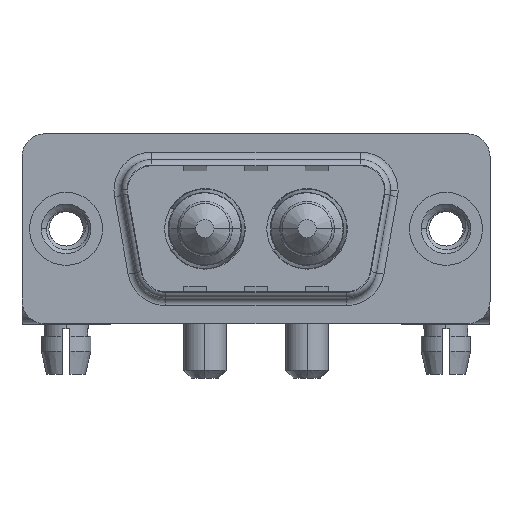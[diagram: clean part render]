
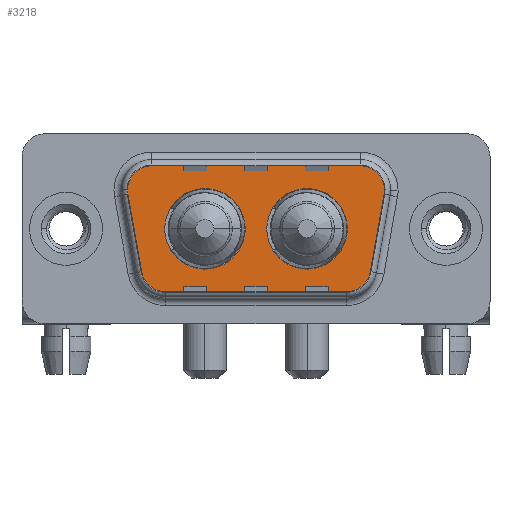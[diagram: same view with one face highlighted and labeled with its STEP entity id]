
A CAD part, top view. The second image highlights one B-rep face of the part: STEP entity #3218.
In plain terms, the highlighted planar face has unit normal (0, 0, 1).
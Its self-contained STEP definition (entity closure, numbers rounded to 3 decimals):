
#93 = ORIENTED_EDGE ( 'NONE', *, *, #6809, .T. ) ;
#292 = EDGE_CURVE ( 'NONE', #4392, #8052, #645, .T. ) ;
#318 = VECTOR ( 'NONE', #12511, 1000. ) ;
#425 = AXIS2_PLACEMENT_3D ( 'NONE', #1729, #8569, #3206 ) ;
#520 = EDGE_CURVE ( 'NONE', #8263, #11774, #11003, .T. ) ;
#546 = CARTESIAN_POINT ( 'NONE',  ( 6.459, -4.9, 0. ) ) ;
#645 = CIRCLE ( 'NONE', #7865, 2. ) ;
#710 = CARTESIAN_POINT ( 'NONE',  ( 19.564, 4.9, 0. ) ) ;
#712 = CARTESIAN_POINT ( 'NONE',  ( 5.436, 4.9, 0. ) ) ;
#745 = DIRECTION ( 'NONE',  ( 0., 0., 1. ) ) ;
#766 = AXIS2_PLACEMENT_3D ( 'NONE', #2552, #10178, #11172 ) ;
#946 = DIRECTION ( 'NONE',  ( 1., 0., 0. ) ) ;
#958 = CARTESIAN_POINT ( 'NONE',  ( 3.466, 2.553, 0. ) ) ;
#1144 = AXIS2_PLACEMENT_3D ( 'NONE', #13453, #7114, #12419 ) ;
#1146 = VECTOR ( 'NONE', #11630, 1000. ) ;
#1548 = CIRCLE ( 'NONE', #425, 2.65 ) ;
#1671 = DIRECTION ( 'NONE',  ( -1., 0., 0. ) ) ;
#1729 = CARTESIAN_POINT ( 'NONE',  ( 9.14, 0., 0. ) ) ;
#2175 = DIRECTION ( 'NONE',  ( 0.174, 0.985, 0. ) ) ;
#2304 = CARTESIAN_POINT ( 'NONE',  ( 21.564, 2.9, 0. ) ) ;
#2376 = LINE ( 'NONE', #5750, #10346 ) ;
#2386 = LINE ( 'NONE', #6473, #11758 ) ;
#2420 = ORIENTED_EDGE ( 'NONE', *, *, #4093, .F. ) ;
#2552 = CARTESIAN_POINT ( 'NONE',  ( 19.564, 2.9, 0. ) ) ;
#2633 = EDGE_LOOP ( 'NONE', ( #11401, #3628 ) ) ;
#3144 = AXIS2_PLACEMENT_3D ( 'NONE', #7506, #10627, #946 ) ;
#3206 = DIRECTION ( 'NONE',  ( 1., 0., 0. ) ) ;
#3218 = ADVANCED_FACE ( 'NONE', ( #9604, #5371, #6571 ), #3320, .T. ) ;
#3296 = CARTESIAN_POINT ( 'NONE',  ( 19.564, 2.9, 0. ) ) ;
#3320 = PLANE ( 'NONE',  #8345 ) ;
#3398 = DIRECTION ( 'NONE',  ( 0., 0., 1. ) ) ;
#3628 = ORIENTED_EDGE ( 'NONE', *, *, #4674, .F. ) ;
#3657 = EDGE_CURVE ( 'NONE', #7756, #6513, #9692, .T. ) ;
#3659 = ORIENTED_EDGE ( 'NONE', *, *, #520, .T. ) ;
#3687 = LINE ( 'NONE', #712, #318 ) ;
#3720 = ORIENTED_EDGE ( 'NONE', *, *, #6664, .T. ) ;
#3819 = ORIENTED_EDGE ( 'NONE', *, *, #4346, .T. ) ;
#4093 = EDGE_CURVE ( 'NONE', #10286, #13687, #13532, .T. ) ;
#4158 = DIRECTION ( 'NONE',  ( 0., 0., 1. ) ) ;
#4346 = EDGE_CURVE ( 'NONE', #11774, #12296, #2376, .T. ) ;
#4392 = VERTEX_POINT ( 'NONE', #2304 ) ;
#4395 = CARTESIAN_POINT ( 'NONE',  ( 5.436, 4.9, 0. ) ) ;
#4599 = EDGE_CURVE ( 'NONE', #6779, #8497, #1548, .T. ) ;
#4674 = EDGE_CURVE ( 'NONE', #8497, #6779, #7204, .T. ) ;
#5371 = FACE_BOUND ( 'NONE', #2633, .T. ) ;
#5428 = CARTESIAN_POINT ( 'NONE',  ( 15.86, 0., 0. ) ) ;
#5509 = CARTESIAN_POINT ( 'NONE',  ( 18.541, -2.9, 0. ) ) ;
#5637 = EDGE_CURVE ( 'NONE', #12296, #7199, #6050, .T. ) ;
#5750 = CARTESIAN_POINT ( 'NONE',  ( 6.459, -4.9, 0. ) ) ;
#5956 = EDGE_LOOP ( 'NONE', ( #7583, #11027, #93, #13091, #3720, #5967, #11973, #3659, #3819 ) ) ;
#5967 = ORIENTED_EDGE ( 'NONE', *, *, #3657, .T. ) ;
#6050 = CIRCLE ( 'NONE', #8752, 2. ) ;
#6413 = DIRECTION ( 'NONE',  ( 0., 0., 1. ) ) ;
#6473 = CARTESIAN_POINT ( 'NONE',  ( 21.534, 2.553, 0. ) ) ;
#6513 = VERTEX_POINT ( 'NONE', #11096 ) ;
#6571 = FACE_OUTER_BOUND ( 'NONE', #5956, .T. ) ;
#6664 = EDGE_CURVE ( 'NONE', #8052, #7756, #3687, .T. ) ;
#6700 = ORIENTED_EDGE ( 'NONE', *, *, #13889, .F. ) ;
#6779 = VERTEX_POINT ( 'NONE', #8062 ) ;
#6809 = EDGE_CURVE ( 'NONE', #11871, #4392, #9328, .T. ) ;
#6915 = CARTESIAN_POINT ( 'NONE',  ( 13.21, 0., 0. ) ) ;
#7114 = DIRECTION ( 'NONE',  ( 0., 0., 1. ) ) ;
#7181 = CARTESIAN_POINT ( 'NONE',  ( 21.534, 2.553, 0. ) ) ;
#7199 = VERTEX_POINT ( 'NONE', #11219 ) ;
#7204 = CIRCLE ( 'NONE', #3144, 2.65 ) ;
#7318 = LINE ( 'NONE', #958, #1146 ) ;
#7506 = CARTESIAN_POINT ( 'NONE',  ( 9.14, 0., 0. ) ) ;
#7583 = ORIENTED_EDGE ( 'NONE', *, *, #5637, .T. ) ;
#7756 = VERTEX_POINT ( 'NONE', #4395 ) ;
#7865 = AXIS2_PLACEMENT_3D ( 'NONE', #3296, #4158, #8591 ) ;
#7957 = DIRECTION ( 'NONE',  ( 1., 0., 0. ) ) ;
#8052 = VERTEX_POINT ( 'NONE', #710 ) ;
#8062 = CARTESIAN_POINT ( 'NONE',  ( 11.79, 0., 0. ) ) ;
#8263 = VERTEX_POINT ( 'NONE', #12713 ) ;
#8300 = AXIS2_PLACEMENT_3D ( 'NONE', #11349, #745, #1671 ) ;
#8345 = AXIS2_PLACEMENT_3D ( 'NONE', #5509, #3398, #10738 ) ;
#8497 = VERTEX_POINT ( 'NONE', #8669 ) ;
#8569 = DIRECTION ( 'NONE',  ( 0., 0., 1. ) ) ;
#8591 = DIRECTION ( 'NONE',  ( -1., 0., 0. ) ) ;
#8669 = CARTESIAN_POINT ( 'NONE',  ( 6.49, 0., 0. ) ) ;
#8752 = AXIS2_PLACEMENT_3D ( 'NONE', #8800, #9928, #7957 ) ;
#8800 = CARTESIAN_POINT ( 'NONE',  ( 18.541, -2.9, 0. ) ) ;
#9103 = AXIS2_PLACEMENT_3D ( 'NONE', #5428, #6413, #10863 ) ;
#9121 = EDGE_LOOP ( 'NONE', ( #2420, #6700 ) ) ;
#9328 = CIRCLE ( 'NONE', #766, 2. ) ;
#9377 = CARTESIAN_POINT ( 'NONE',  ( 5.436, 2.9, 0. ) ) ;
#9604 = FACE_BOUND ( 'NONE', #9121, .T. ) ;
#9692 = CIRCLE ( 'NONE', #11505, 2. ) ;
#9928 = DIRECTION ( 'NONE',  ( 0., 0., 1. ) ) ;
#10064 = DIRECTION ( 'NONE',  ( 1., 0., 0. ) ) ;
#10178 = DIRECTION ( 'NONE',  ( 0., 0., 1. ) ) ;
#10240 = DIRECTION ( 'NONE',  ( 0., 0., 1. ) ) ;
#10286 = VERTEX_POINT ( 'NONE', #10312 ) ;
#10312 = CARTESIAN_POINT ( 'NONE',  ( 18.51, 0., 0. ) ) ;
#10346 = VECTOR ( 'NONE', #10064, 1000. ) ;
#10627 = DIRECTION ( 'NONE',  ( 0., 0., 1. ) ) ;
#10738 = DIRECTION ( 'NONE',  ( 1., 0., 0. ) ) ;
#10863 = DIRECTION ( 'NONE',  ( 1., 0., 0. ) ) ;
#11003 = CIRCLE ( 'NONE', #8300, 2. ) ;
#11027 = ORIENTED_EDGE ( 'NONE', *, *, #11637, .T. ) ;
#11096 = CARTESIAN_POINT ( 'NONE',  ( 3.466, 2.553, 0. ) ) ;
#11172 = DIRECTION ( 'NONE',  ( -1., 0., 0. ) ) ;
#11219 = CARTESIAN_POINT ( 'NONE',  ( 20.511, -3.247, 0. ) ) ;
#11349 = CARTESIAN_POINT ( 'NONE',  ( 6.459, -2.9, 0. ) ) ;
#11401 = ORIENTED_EDGE ( 'NONE', *, *, #4599, .F. ) ;
#11473 = CARTESIAN_POINT ( 'NONE',  ( 18.541, -4.9, 0. ) ) ;
#11505 = AXIS2_PLACEMENT_3D ( 'NONE', #9377, #10240, #12432 ) ;
#11630 = DIRECTION ( 'NONE',  ( 0.174, -0.985, 0. ) ) ;
#11637 = EDGE_CURVE ( 'NONE', #7199, #11871, #2386, .T. ) ;
#11758 = VECTOR ( 'NONE', #2175, 1000. ) ;
#11774 = VERTEX_POINT ( 'NONE', #546 ) ;
#11855 = EDGE_CURVE ( 'NONE', #6513, #8263, #7318, .T. ) ;
#11871 = VERTEX_POINT ( 'NONE', #7181 ) ;
#11973 = ORIENTED_EDGE ( 'NONE', *, *, #11855, .T. ) ;
#12296 = VERTEX_POINT ( 'NONE', #11473 ) ;
#12419 = DIRECTION ( 'NONE',  ( 1., 0., 0. ) ) ;
#12432 = DIRECTION ( 'NONE',  ( 1., 0., 0. ) ) ;
#12511 = DIRECTION ( 'NONE',  ( -1., 0., 0. ) ) ;
#12713 = CARTESIAN_POINT ( 'NONE',  ( 4.489, -3.247, 0. ) ) ;
#13091 = ORIENTED_EDGE ( 'NONE', *, *, #292, .T. ) ;
#13150 = CIRCLE ( 'NONE', #9103, 2.65 ) ;
#13453 = CARTESIAN_POINT ( 'NONE',  ( 15.86, 0., 0. ) ) ;
#13532 = CIRCLE ( 'NONE', #1144, 2.65 ) ;
#13687 = VERTEX_POINT ( 'NONE', #6915 ) ;
#13889 = EDGE_CURVE ( 'NONE', #13687, #10286, #13150, .T. ) ;
